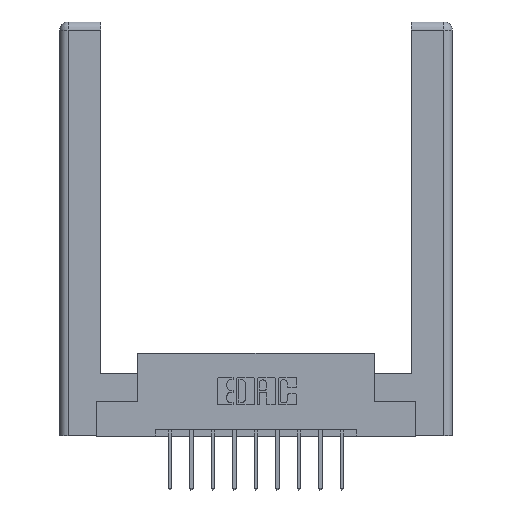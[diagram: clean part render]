
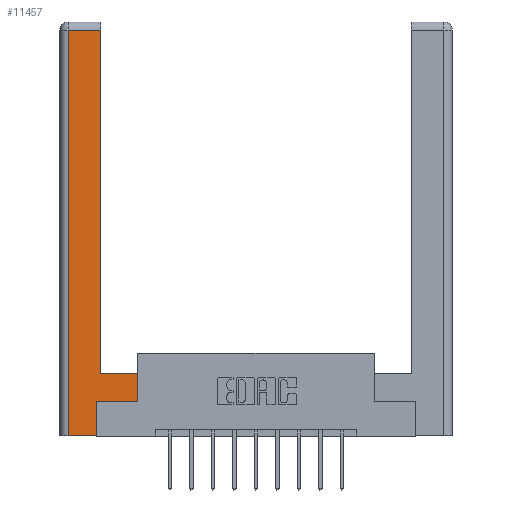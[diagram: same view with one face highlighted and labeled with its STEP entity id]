
A CAD part, top view. The second image highlights one B-rep face of the part: STEP entity #11457.
In plain terms, the highlighted planar face has unit normal (0, 0, 1).
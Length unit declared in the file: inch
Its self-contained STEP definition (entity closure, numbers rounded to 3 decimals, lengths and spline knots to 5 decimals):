
#282 = ORIENTED_EDGE ( 'NONE', *, *, #2368, .T. ) ;
#522 = AXIS2_PLACEMENT_3D ( 'NONE', #10814, #8562, #4328 ) ;
#861 = VECTOR ( 'NONE', #13712, 39.37008 ) ;
#971 = VERTEX_POINT ( 'NONE', #3381 ) ;
#1036 = CARTESIAN_POINT ( 'NONE',  ( 0.0615, 0., 0. ) ) ;
#1061 = VERTEX_POINT ( 'NONE', #1200 ) ;
#1200 = CARTESIAN_POINT ( 'NONE',  ( 0.265, 0., 0. ) ) ;
#1470 = VECTOR ( 'NONE', #12269, 39.37008 ) ;
#1618 = CARTESIAN_POINT ( 'NONE',  ( 0.565, 0.245, 0. ) ) ;
#1712 = ORIENTED_EDGE ( 'NONE', *, *, #7135, .T. ) ;
#2001 = CARTESIAN_POINT ( 'NONE',  ( 0.565, 0.45, 0. ) ) ;
#2102 = VECTOR ( 'NONE', #13288, 39.37008 ) ;
#2368 = EDGE_CURVE ( 'NONE', #1061, #971, #5907, .T. ) ;
#2898 = VECTOR ( 'NONE', #12174, 39.37008 ) ;
#3066 = VECTOR ( 'NONE', #3175, 39.37008 ) ;
#3123 = FACE_OUTER_BOUND ( 'NONE', #7106, .T. ) ;
#3175 = DIRECTION ( 'NONE',  ( 0., 1., 0. ) ) ;
#3216 = ORIENTED_EDGE ( 'NONE', *, *, #10822, .T. ) ;
#3381 = CARTESIAN_POINT ( 'NONE',  ( 0.265, 0.245, 0. ) ) ;
#4042 = CARTESIAN_POINT ( 'NONE',  ( 0.295, 3., 0. ) ) ;
#4044 = DIRECTION ( 'NONE',  ( -1., 0., 0. ) ) ;
#4328 = DIRECTION ( 'NONE',  ( -1., 0., 0. ) ) ;
#4340 = ORIENTED_EDGE ( 'NONE', *, *, #5641, .T. ) ;
#4678 = CARTESIAN_POINT ( 'NONE',  ( 0.565, 0.45, 0. ) ) ;
#4982 = VERTEX_POINT ( 'NONE', #2001 ) ;
#5641 = EDGE_CURVE ( 'NONE', #971, #8972, #11751, .T. ) ;
#5907 = LINE ( 'NONE', #6370, #3066 ) ;
#5989 = LINE ( 'NONE', #4678, #8213 ) ;
#6177 = PLANE ( 'NONE',  #522 ) ;
#6370 = CARTESIAN_POINT ( 'NONE',  ( 0.265, 0.245, 0. ) ) ;
#7053 = VERTEX_POINT ( 'NONE', #12705 ) ;
#7106 = EDGE_LOOP ( 'NONE', ( #1712, #11078, #3216, #10277, #282, #4340, #11231, #10834 ) ) ;
#7135 = EDGE_CURVE ( 'NONE', #10302, #7053, #7984, .T. ) ;
#7224 = LINE ( 'NONE', #12708, #9912 ) ;
#7592 = EDGE_CURVE ( 'NONE', #7926, #1061, #9334, .T. ) ;
#7926 = VERTEX_POINT ( 'NONE', #1036 ) ;
#7984 = LINE ( 'NONE', #4042, #861 ) ;
#8213 = VECTOR ( 'NONE', #11206, 39.37008 ) ;
#8290 = LINE ( 'NONE', #10380, #10473 ) ;
#8562 = DIRECTION ( 'NONE',  ( 0., 0., -1. ) ) ;
#8972 = VERTEX_POINT ( 'NONE', #10119 ) ;
#9334 = LINE ( 'NONE', #9928, #2898 ) ;
#9912 = VECTOR ( 'NONE', #4044, 39.37008 ) ;
#9928 = CARTESIAN_POINT ( 'NONE',  ( 0.265, 0., 0. ) ) ;
#10025 = EDGE_CURVE ( 'NONE', #4982, #10302, #7224, .T. ) ;
#10119 = CARTESIAN_POINT ( 'NONE',  ( 0.565, 0.245, 0. ) ) ;
#10277 = ORIENTED_EDGE ( 'NONE', *, *, #7592, .T. ) ;
#10302 = VERTEX_POINT ( 'NONE', #12536 ) ;
#10380 = CARTESIAN_POINT ( 'NONE',  ( 0.0615, 2.94, 0. ) ) ;
#10473 = VECTOR ( 'NONE', #12530, 39.37008 ) ;
#10558 = EDGE_CURVE ( 'NONE', #8972, #4982, #5989, .T. ) ;
#10814 = CARTESIAN_POINT ( 'NONE',  ( 0., 0., 0. ) ) ;
#10822 = EDGE_CURVE ( 'NONE', #12457, #7926, #13223, .T. ) ;
#10834 = ORIENTED_EDGE ( 'NONE', *, *, #10025, .T. ) ;
#11042 = CARTESIAN_POINT ( 'NONE',  ( 0.0615, 2.94, 0. ) ) ;
#11078 = ORIENTED_EDGE ( 'NONE', *, *, #12919, .T. ) ;
#11206 = DIRECTION ( 'NONE',  ( 0., 1., 0. ) ) ;
#11231 = ORIENTED_EDGE ( 'NONE', *, *, #10558, .T. ) ;
#11457 = ADVANCED_FACE ( 'NONE', ( #3123 ), #6177, .F. ) ;
#11751 = LINE ( 'NONE', #1618, #1470 ) ;
#12174 = DIRECTION ( 'NONE',  ( 1., 0., 0. ) ) ;
#12225 = CARTESIAN_POINT ( 'NONE',  ( 0.0615, 0., 0. ) ) ;
#12269 = DIRECTION ( 'NONE',  ( 1., 0., 0. ) ) ;
#12457 = VERTEX_POINT ( 'NONE', #11042 ) ;
#12530 = DIRECTION ( 'NONE',  ( -1., 0., 0. ) ) ;
#12536 = CARTESIAN_POINT ( 'NONE',  ( 0.295, 0.45, 0. ) ) ;
#12705 = CARTESIAN_POINT ( 'NONE',  ( 0.295, 2.94, 0. ) ) ;
#12708 = CARTESIAN_POINT ( 'NONE',  ( 0.295, 0.45, 0. ) ) ;
#12919 = EDGE_CURVE ( 'NONE', #7053, #12457, #8290, .T. ) ;
#13223 = LINE ( 'NONE', #12225, #2102 ) ;
#13288 = DIRECTION ( 'NONE',  ( 0., -1., 0. ) ) ;
#13712 = DIRECTION ( 'NONE',  ( 0., 1., 0. ) ) ;
